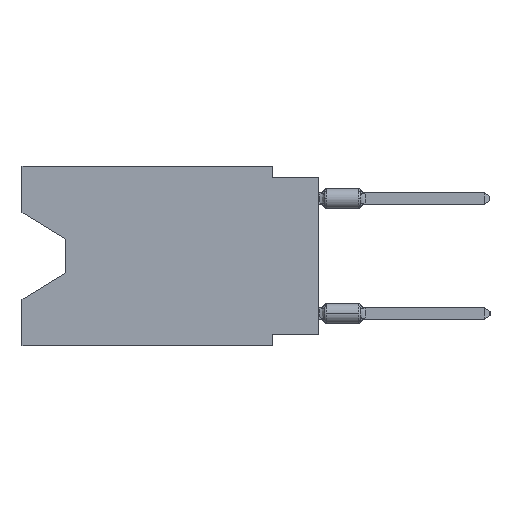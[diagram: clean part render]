
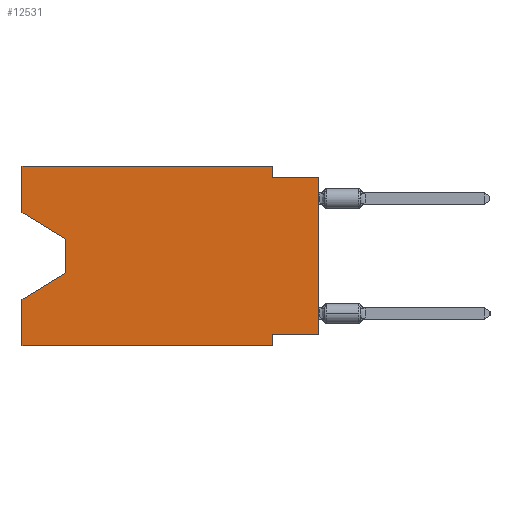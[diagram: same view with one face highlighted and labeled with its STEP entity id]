
A CAD part, left-side view. The second image highlights one B-rep face of the part: STEP entity #12531.
In plain terms, the highlighted planar face has unit normal (-1, 0, 0).
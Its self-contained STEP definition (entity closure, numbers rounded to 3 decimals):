
#545 = LINE ( 'NONE', #12506, #2131 ) ;
#723 = DIRECTION ( 'NONE',  ( 0., 0., -1. ) ) ;
#919 = EDGE_CURVE ( 'NONE', #29410, #17161, #36028, .T. ) ;
#1065 = CARTESIAN_POINT ( 'NONE',  ( 0., 16.383, -2.546 ) ) ;
#1571 = EDGE_CURVE ( 'NONE', #32780, #17161, #6807, .T. ) ;
#1877 = PLANE ( 'NONE',  #16395 ) ;
#2079 = ORIENTED_EDGE ( 'NONE', *, *, #37457, .F. ) ;
#2131 = VECTOR ( 'NONE', #27801, 1000. ) ;
#2269 = VECTOR ( 'NONE', #33516, 1000. ) ;
#2691 = DIRECTION ( 'NONE',  ( 0., 0., -1. ) ) ;
#3597 = CARTESIAN_POINT ( 'NONE',  ( 0., 16.383, -9.906 ) ) ;
#4487 = ORIENTED_EDGE ( 'NONE', *, *, #1571, .F. ) ;
#5492 = CARTESIAN_POINT ( 'NONE',  ( 0., 0., -9.271 ) ) ;
#6440 = ORIENTED_EDGE ( 'NONE', *, *, #29264, .F. ) ;
#6807 = LINE ( 'NONE', #18019, #31136 ) ;
#7233 = CARTESIAN_POINT ( 'NONE',  ( 0., 16.383, -2.546 ) ) ;
#7373 = CARTESIAN_POINT ( 'NONE',  ( 0., 0., -0.635 ) ) ;
#8199 = DIRECTION ( 'NONE',  ( 0., 0.855, -0.519 ) ) ;
#8577 = LINE ( 'NONE', #26741, #10449 ) ;
#8662 = LINE ( 'NONE', #23185, #18736 ) ;
#9462 = VECTOR ( 'NONE', #723, 1000. ) ;
#9505 = ORIENTED_EDGE ( 'NONE', *, *, #28550, .F. ) ;
#9536 = VECTOR ( 'NONE', #37562, 1000. ) ;
#10449 = VECTOR ( 'NONE', #32360, 1000. ) ;
#11459 = VECTOR ( 'NONE', #8199, 1000. ) ;
#12506 = CARTESIAN_POINT ( 'NONE',  ( 0., 16.383, -9.906 ) ) ;
#12531 = ADVANCED_FACE ( 'NONE', ( #16572 ), #1877, .F. ) ;
#12808 = DIRECTION ( 'NONE',  ( 0., 0., 1. ) ) ;
#13764 = ORIENTED_EDGE ( 'NONE', *, *, #16810, .F. ) ;
#14065 = EDGE_CURVE ( 'NONE', #35828, #29384, #15927, .T. ) ;
#14627 = CARTESIAN_POINT ( 'NONE',  ( 0., 0., -9.271 ) ) ;
#14696 = VECTOR ( 'NONE', #12808, 1000. ) ;
#15318 = DIRECTION ( 'NONE',  ( 0., -1., 0. ) ) ;
#15328 = VECTOR ( 'NONE', #32168, 1000. ) ;
#15340 = CARTESIAN_POINT ( 'NONE',  ( 0., 2.54, -0.635 ) ) ;
#15407 = LINE ( 'NONE', #27211, #9462 ) ;
#15508 = ORIENTED_EDGE ( 'NONE', *, *, #14065, .T. ) ;
#15719 = CARTESIAN_POINT ( 'NONE',  ( 0., 0., 0. ) ) ;
#15927 = LINE ( 'NONE', #7233, #2269 ) ;
#16332 = ORIENTED_EDGE ( 'NONE', *, *, #20216, .F. ) ;
#16395 = AXIS2_PLACEMENT_3D ( 'NONE', #28005, #25281, #18911 ) ;
#16498 = LINE ( 'NONE', #19961, #9536 ) ;
#16572 = FACE_OUTER_BOUND ( 'NONE', #26698, .T. ) ;
#16574 = DIRECTION ( 'NONE',  ( 0., 0., -1. ) ) ;
#16810 = EDGE_CURVE ( 'NONE', #35828, #19615, #16498, .T. ) ;
#17161 = VERTEX_POINT ( 'NONE', #7373 ) ;
#17319 = CARTESIAN_POINT ( 'NONE',  ( 0., 16.383, 0. ) ) ;
#18019 = CARTESIAN_POINT ( 'NONE',  ( 0., 0., -0.635 ) ) ;
#18089 = CARTESIAN_POINT ( 'NONE',  ( 0., 13.97, -5.893 ) ) ;
#18526 = ORIENTED_EDGE ( 'NONE', *, *, #26775, .T. ) ;
#18736 = VECTOR ( 'NONE', #2691, 1000. ) ;
#18911 = DIRECTION ( 'NONE',  ( 0., 0., -1. ) ) ;
#19063 = VECTOR ( 'NONE', #22561, 1000. ) ;
#19274 = LINE ( 'NONE', #5492, #15328 ) ;
#19458 = LINE ( 'NONE', #17319, #19063 ) ;
#19615 = VERTEX_POINT ( 'NONE', #22088 ) ;
#19961 = CARTESIAN_POINT ( 'NONE',  ( 0., 16.383, 0. ) ) ;
#20216 = EDGE_CURVE ( 'NONE', #33469, #37401, #8662, .T. ) ;
#20930 = ORIENTED_EDGE ( 'NONE', *, *, #919, .T. ) ;
#22088 = CARTESIAN_POINT ( 'NONE',  ( 0., 16.383, 0. ) ) ;
#22499 = EDGE_CURVE ( 'NONE', #22894, #37401, #545, .T. ) ;
#22561 = DIRECTION ( 'NONE',  ( 0., -1., 0. ) ) ;
#22563 = VERTEX_POINT ( 'NONE', #25658 ) ;
#22894 = VERTEX_POINT ( 'NONE', #3597 ) ;
#23185 = CARTESIAN_POINT ( 'NONE',  ( 0., 2.54, -9.906 ) ) ;
#24126 = VERTEX_POINT ( 'NONE', #18089 ) ;
#24326 = EDGE_CURVE ( 'NONE', #24126, #22563, #26563, .T. ) ;
#25281 = DIRECTION ( 'NONE',  ( 1., 0., 0. ) ) ;
#25327 = VERTEX_POINT ( 'NONE', #36913 ) ;
#25468 = LINE ( 'NONE', #36507, #35729 ) ;
#25658 = CARTESIAN_POINT ( 'NONE',  ( 0., 16.383, -7.36 ) ) ;
#25861 = CARTESIAN_POINT ( 'NONE',  ( 0., 13.97, -4.013 ) ) ;
#26302 = CARTESIAN_POINT ( 'NONE',  ( 0., 2.54, -9.271 ) ) ;
#26459 = ORIENTED_EDGE ( 'NONE', *, *, #24326, .T. ) ;
#26563 = LINE ( 'NONE', #31991, #11459 ) ;
#26698 = EDGE_LOOP ( 'NONE', ( #15508, #18526, #26459, #30208, #37462, #16332, #9505, #20930, #4487, #6440, #2079, #13764 ) ) ;
#26741 = CARTESIAN_POINT ( 'NONE',  ( 0., 16.383, 0. ) ) ;
#26775 = EDGE_CURVE ( 'NONE', #29384, #24126, #15407, .T. ) ;
#27211 = CARTESIAN_POINT ( 'NONE',  ( 0., 13.97, -4.013 ) ) ;
#27801 = DIRECTION ( 'NONE',  ( 0., -1., 0. ) ) ;
#28005 = CARTESIAN_POINT ( 'NONE',  ( 0., 16.383, 0. ) ) ;
#28550 = EDGE_CURVE ( 'NONE', #29410, #33469, #19274, .T. ) ;
#29264 = EDGE_CURVE ( 'NONE', #25327, #32780, #25468, .T. ) ;
#29384 = VERTEX_POINT ( 'NONE', #25861 ) ;
#29410 = VERTEX_POINT ( 'NONE', #14627 ) ;
#30208 = ORIENTED_EDGE ( 'NONE', *, *, #38107, .F. ) ;
#31136 = VECTOR ( 'NONE', #15318, 1000. ) ;
#31991 = CARTESIAN_POINT ( 'NONE',  ( 0., 13.97, -5.893 ) ) ;
#32168 = DIRECTION ( 'NONE',  ( 0., 1., 0. ) ) ;
#32360 = DIRECTION ( 'NONE',  ( 0., 0., 1. ) ) ;
#32780 = VERTEX_POINT ( 'NONE', #15340 ) ;
#33469 = VERTEX_POINT ( 'NONE', #26302 ) ;
#33516 = DIRECTION ( 'NONE',  ( 0., -0.855, -0.519 ) ) ;
#35729 = VECTOR ( 'NONE', #16574, 1000. ) ;
#35775 = CARTESIAN_POINT ( 'NONE',  ( 0., 2.54, -9.906 ) ) ;
#35828 = VERTEX_POINT ( 'NONE', #1065 ) ;
#36028 = LINE ( 'NONE', #15719, #14696 ) ;
#36507 = CARTESIAN_POINT ( 'NONE',  ( 0., 2.54, 0. ) ) ;
#36913 = CARTESIAN_POINT ( 'NONE',  ( 0., 2.54, 0. ) ) ;
#37401 = VERTEX_POINT ( 'NONE', #35775 ) ;
#37457 = EDGE_CURVE ( 'NONE', #19615, #25327, #19458, .T. ) ;
#37462 = ORIENTED_EDGE ( 'NONE', *, *, #22499, .T. ) ;
#37562 = DIRECTION ( 'NONE',  ( 0., 0., 1. ) ) ;
#38107 = EDGE_CURVE ( 'NONE', #22894, #22563, #8577, .T. ) ;
